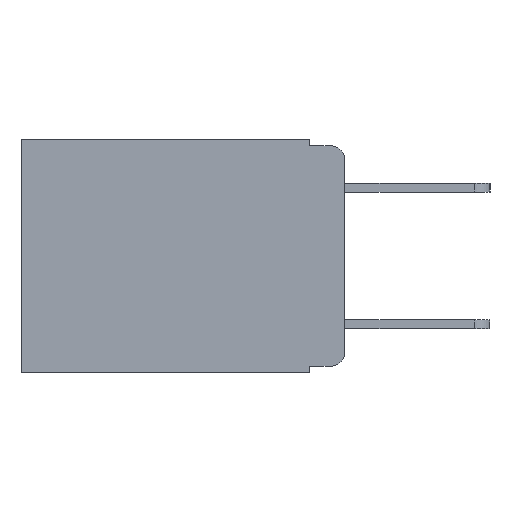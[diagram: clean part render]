
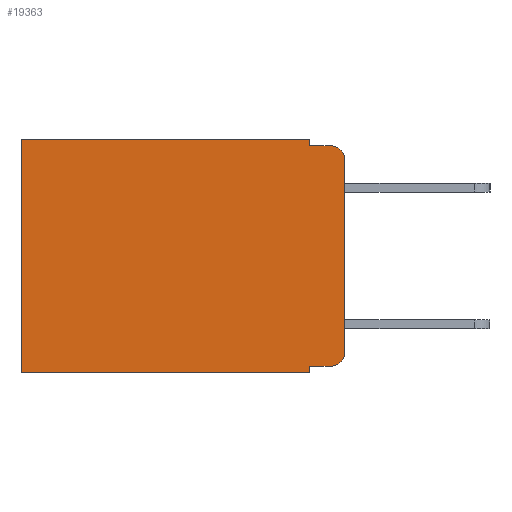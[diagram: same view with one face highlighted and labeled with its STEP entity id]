
A CAD part, left-side view. The second image highlights one B-rep face of the part: STEP entity #19363.
In plain terms, the highlighted planar face has unit normal (-1, 0, 0).
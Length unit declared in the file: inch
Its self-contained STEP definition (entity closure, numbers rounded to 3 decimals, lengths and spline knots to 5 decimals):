
#184 = CARTESIAN_POINT ( 'NONE',  ( 0.298, 0.473, -0.343 ) ) ;
#314 = VECTOR ( 'NONE', #475, 39.37008 ) ;
#410 = EDGE_CURVE ( 'NONE', #9875, #1377, #17210, .T. ) ;
#475 = DIRECTION ( 'NONE',  ( 0., -1., 0. ) ) ;
#657 = ORIENTED_EDGE ( 'NONE', *, *, #17282, .F. ) ;
#670 = ORIENTED_EDGE ( 'NONE', *, *, #14271, .T. ) ;
#700 = ORIENTED_EDGE ( 'NONE', *, *, #20117, .F. ) ;
#746 = ORIENTED_EDGE ( 'NONE', *, *, #20219, .F. ) ;
#849 = ORIENTED_EDGE ( 'NONE', *, *, #2528, .T. ) ;
#1111 = ORIENTED_EDGE ( 'NONE', *, *, #410, .T. ) ;
#1311 = DIRECTION ( 'NONE',  ( 0., 0., -1. ) ) ;
#1377 = VERTEX_POINT ( 'NONE', #184 ) ;
#1445 = VECTOR ( 'NONE', #14685, 39.37008 ) ;
#1471 = ORIENTED_EDGE ( 'NONE', *, *, #6325, .F. ) ;
#1487 = CARTESIAN_POINT ( 'NONE',  ( 0.298, 0., -0.313 ) ) ;
#1501 = ORIENTED_EDGE ( 'NONE', *, *, #3230, .F. ) ;
#1609 = LINE ( 'NONE', #14865, #4818 ) ;
#1616 = VERTEX_POINT ( 'NONE', #11638 ) ;
#1695 = ORIENTED_EDGE ( 'NONE', *, *, #17903, .T. ) ;
#1766 = ORIENTED_EDGE ( 'NONE', *, *, #11837, .T. ) ;
#1829 = VERTEX_POINT ( 'NONE', #7097 ) ;
#2528 = EDGE_CURVE ( 'NONE', #7664, #9875, #13516, .T. ) ;
#2568 = VECTOR ( 'NONE', #4939, 39.37008 ) ;
#3057 = LINE ( 'NONE', #18620, #1445 ) ;
#3230 = EDGE_CURVE ( 'NONE', #19796, #1829, #13241, .T. ) ;
#3576 = CARTESIAN_POINT ( 'NONE',  ( 0.298, 0., 0. ) ) ;
#4007 = DIRECTION ( 'NONE',  ( 0., 0., -1. ) ) ;
#4018 = DIRECTION ( 'NONE',  ( -1., 0., 0. ) ) ;
#4415 = LINE ( 'NONE', #17661, #8229 ) ;
#4558 = CIRCLE ( 'NONE', #13251, 0.02 ) ;
#4818 = VECTOR ( 'NONE', #16354, 39.37008 ) ;
#4939 = DIRECTION ( 'NONE',  ( 0., -1., 0. ) ) ;
#5066 = EDGE_LOOP ( 'NONE', ( #657, #670, #700, #746, #849, #1111, #1471, #1501, #1695, #1766 ) ) ;
#5302 = CARTESIAN_POINT ( 'NONE',  ( 0.298, 0.02, -0.333 ) ) ;
#5309 = VERTEX_POINT ( 'NONE', #1487 ) ;
#5684 = CARTESIAN_POINT ( 'NONE',  ( 0.298, 0.051, -0.333 ) ) ;
#6325 = EDGE_CURVE ( 'NONE', #1829, #1377, #3057, .T. ) ;
#7097 = CARTESIAN_POINT ( 'NONE',  ( 0.298, 0.051, -0.343 ) ) ;
#7241 = PLANE ( 'NONE',  #11811 ) ;
#7586 = VECTOR ( 'NONE', #16823, 39.37008 ) ;
#7664 = VERTEX_POINT ( 'NONE', #11111 ) ;
#8229 = VECTOR ( 'NONE', #16199, 39.37008 ) ;
#8843 = LINE ( 'NONE', #10626, #314 ) ;
#8876 = CARTESIAN_POINT ( 'NONE',  ( 0.298, 0., 0. ) ) ;
#9181 = CARTESIAN_POINT ( 'NONE',  ( 0.298, 0.051, 0. ) ) ;
#9875 = VERTEX_POINT ( 'NONE', #13539 ) ;
#10138 = CARTESIAN_POINT ( 'NONE',  ( 0.298, 0.02, -0.313 ) ) ;
#10626 = CARTESIAN_POINT ( 'NONE',  ( 0.298, 0.051, -0.333 ) ) ;
#11111 = CARTESIAN_POINT ( 'NONE',  ( 0.298, 0.051, 0. ) ) ;
#11211 = VERTEX_POINT ( 'NONE', #13333 ) ;
#11331 = CARTESIAN_POINT ( 'NONE',  ( 0.298, 0.051, -0.01 ) ) ;
#11638 = CARTESIAN_POINT ( 'NONE',  ( 0.298, 0.051, -0.01 ) ) ;
#11698 = DIRECTION ( 'NONE',  ( 0., 0., -1. ) ) ;
#11811 = AXIS2_PLACEMENT_3D ( 'NONE', #8876, #13591, #4007 ) ;
#11837 = EDGE_CURVE ( 'NONE', #18277, #5309, #4558, .T. ) ;
#12183 = DIRECTION ( 'NONE',  ( 0., 1., 0. ) ) ;
#13241 = LINE ( 'NONE', #9181, #7586 ) ;
#13251 = AXIS2_PLACEMENT_3D ( 'NONE', #10138, #20534, #11698 ) ;
#13333 = CARTESIAN_POINT ( 'NONE',  ( 0.298, 0., -0.03 ) ) ;
#13516 = LINE ( 'NONE', #3576, #20387 ) ;
#13539 = CARTESIAN_POINT ( 'NONE',  ( 0.298, 0.473, 0. ) ) ;
#13591 = DIRECTION ( 'NONE',  ( 1., 0., 0. ) ) ;
#13600 = CARTESIAN_POINT ( 'NONE',  ( 0.298, 0.02, -0.03 ) ) ;
#14256 = CARTESIAN_POINT ( 'NONE',  ( 0.298, 0.02, -0.01 ) ) ;
#14271 = EDGE_CURVE ( 'NONE', #11211, #15643, #20544, .T. ) ;
#14685 = DIRECTION ( 'NONE',  ( 0., 1., 0. ) ) ;
#14865 = CARTESIAN_POINT ( 'NONE',  ( 0.298, 0., 0. ) ) ;
#15141 = DIRECTION ( 'NONE',  ( 0., 0., -1. ) ) ;
#15643 = VERTEX_POINT ( 'NONE', #14256 ) ;
#15788 = LINE ( 'NONE', #11331, #2568 ) ;
#16199 = DIRECTION ( 'NONE',  ( 0., 0., -1. ) ) ;
#16354 = DIRECTION ( 'NONE',  ( 0., 0., -1. ) ) ;
#16823 = DIRECTION ( 'NONE',  ( 0., 0., -1. ) ) ;
#17210 = LINE ( 'NONE', #17709, #17646 ) ;
#17282 = EDGE_CURVE ( 'NONE', #11211, #5309, #1609, .T. ) ;
#17646 = VECTOR ( 'NONE', #1311, 39.37008 ) ;
#17652 = FACE_OUTER_BOUND ( 'NONE', #5066, .T. ) ;
#17661 = CARTESIAN_POINT ( 'NONE',  ( 0.298, 0.051, 0. ) ) ;
#17709 = CARTESIAN_POINT ( 'NONE',  ( 0.298, 0.473, 0. ) ) ;
#17903 = EDGE_CURVE ( 'NONE', #19796, #18277, #8843, .T. ) ;
#18277 = VERTEX_POINT ( 'NONE', #5302 ) ;
#18620 = CARTESIAN_POINT ( 'NONE',  ( 0.298, 0., -0.343 ) ) ;
#18983 = AXIS2_PLACEMENT_3D ( 'NONE', #13600, #4018, #15141 ) ;
#19363 = ADVANCED_FACE ( 'NONE', ( #17652 ), #7241, .F. ) ;
#19796 = VERTEX_POINT ( 'NONE', #5684 ) ;
#20117 = EDGE_CURVE ( 'NONE', #1616, #15643, #15788, .T. ) ;
#20219 = EDGE_CURVE ( 'NONE', #7664, #1616, #4415, .T. ) ;
#20387 = VECTOR ( 'NONE', #12183, 39.37008 ) ;
#20534 = DIRECTION ( 'NONE',  ( -1., 0., 0. ) ) ;
#20544 = CIRCLE ( 'NONE', #18983, 0.02 ) ;
